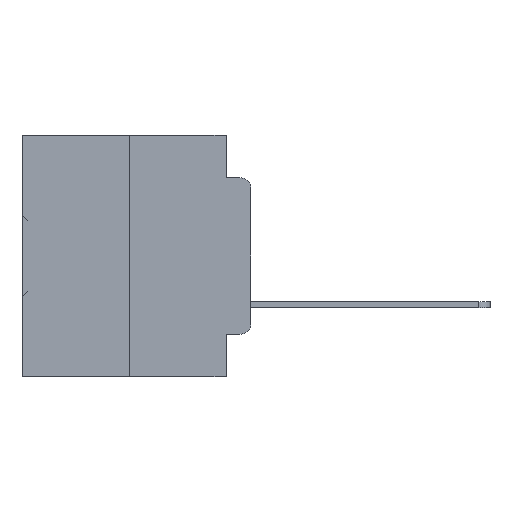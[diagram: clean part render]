
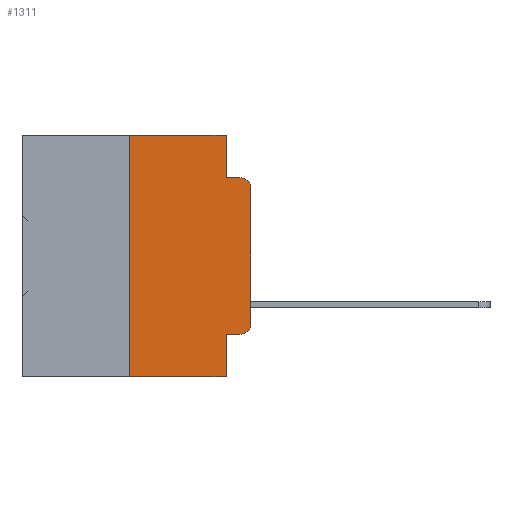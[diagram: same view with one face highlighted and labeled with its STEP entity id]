
A CAD part, left-side view. The second image highlights one B-rep face of the part: STEP entity #1311.
In plain terms, the highlighted planar face has unit normal (-1, 0, 0).
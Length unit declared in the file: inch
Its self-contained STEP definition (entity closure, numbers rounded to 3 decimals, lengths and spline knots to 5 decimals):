
#771 = EDGE_CURVE ( 'NONE', #20657, #15673, #15072, .T. ) ;
#1311 = ADVANCED_FACE ( 'NONE', ( #11215 ), #8687, .F. ) ;
#1824 = LINE ( 'NONE', #27525, #25090 ) ;
#2184 = VECTOR ( 'NONE', #33086, 39.37008 ) ;
#2272 = CARTESIAN_POINT ( 'NONE',  ( 0., 0.051, -0.4115 ) ) ;
#2706 = CARTESIAN_POINT ( 'NONE',  ( 0., 0.051, 0. ) ) ;
#3140 = ORIENTED_EDGE ( 'NONE', *, *, #29928, .T. ) ;
#3907 = VERTEX_POINT ( 'NONE', #31514 ) ;
#4711 = VERTEX_POINT ( 'NONE', #8743 ) ;
#5124 = CARTESIAN_POINT ( 'NONE',  ( 0., 0., -0.1085 ) ) ;
#5289 = CARTESIAN_POINT ( 'NONE',  ( 0., 0.02, -0.1085 ) ) ;
#5407 = ORIENTED_EDGE ( 'NONE', *, *, #12841, .F. ) ;
#5420 = ORIENTED_EDGE ( 'NONE', *, *, #36283, .F. ) ;
#6996 = VECTOR ( 'NONE', #14801, 39.37008 ) ;
#7180 = VECTOR ( 'NONE', #24824, 39.37008 ) ;
#7764 = EDGE_CURVE ( 'NONE', #3907, #27670, #10228, .T. ) ;
#8336 = DIRECTION ( 'NONE',  ( 0., 0., -1. ) ) ;
#8360 = LINE ( 'NONE', #26220, #14506 ) ;
#8659 = ORIENTED_EDGE ( 'NONE', *, *, #31378, .T. ) ;
#8687 = PLANE ( 'NONE',  #10043 ) ;
#8743 = CARTESIAN_POINT ( 'NONE',  ( 0., 0.02, -0.0885 ) ) ;
#9107 = DIRECTION ( 'NONE',  ( 0., -1., 0. ) ) ;
#9382 = VERTEX_POINT ( 'NONE', #32377 ) ;
#9793 = CARTESIAN_POINT ( 'NONE',  ( 0., 0.051, -0.0885 ) ) ;
#10043 = AXIS2_PLACEMENT_3D ( 'NONE', #36058, #17841, #39101 ) ;
#10228 = LINE ( 'NONE', #2706, #2184 ) ;
#11196 = CIRCLE ( 'NONE', #31931, 0.02 ) ;
#11215 = FACE_OUTER_BOUND ( 'NONE', #35360, .T. ) ;
#12841 = EDGE_CURVE ( 'NONE', #13925, #3907, #30212, .T. ) ;
#13925 = VERTEX_POINT ( 'NONE', #16389 ) ;
#14410 = CARTESIAN_POINT ( 'NONE',  ( 0., 0.02, -0.4115 ) ) ;
#14506 = VECTOR ( 'NONE', #20110, 39.37008 ) ;
#14801 = DIRECTION ( 'NONE',  ( 0., 0., -1. ) ) ;
#15072 = LINE ( 'NONE', #26926, #6996 ) ;
#15083 = CARTESIAN_POINT ( 'NONE',  ( 0., 0.473, -0.5 ) ) ;
#15673 = VERTEX_POINT ( 'NONE', #33550 ) ;
#16389 = CARTESIAN_POINT ( 'NONE',  ( 0., 0.25, 0. ) ) ;
#16732 = AXIS2_PLACEMENT_3D ( 'NONE', #35150, #16921, #38180 ) ;
#16921 = DIRECTION ( 'NONE',  ( -1., 0., 0. ) ) ;
#17728 = EDGE_CURVE ( 'NONE', #9382, #21263, #1824, .T. ) ;
#17841 = DIRECTION ( 'NONE',  ( 1., 0., 0. ) ) ;
#18744 = ORIENTED_EDGE ( 'NONE', *, *, #18811, .F. ) ;
#18811 = EDGE_CURVE ( 'NONE', #24144, #13925, #8360, .T. ) ;
#20110 = DIRECTION ( 'NONE',  ( 0., 0., 1. ) ) ;
#20512 = DIRECTION ( 'NONE',  ( 0., -1., 0. ) ) ;
#20615 = VECTOR ( 'NONE', #22107, 39.37008 ) ;
#20657 = VERTEX_POINT ( 'NONE', #2272 ) ;
#21263 = VERTEX_POINT ( 'NONE', #5124 ) ;
#21913 = CIRCLE ( 'NONE', #16732, 0.02 ) ;
#22107 = DIRECTION ( 'NONE',  ( 0., -1., 0. ) ) ;
#24144 = VERTEX_POINT ( 'NONE', #24286 ) ;
#24286 = CARTESIAN_POINT ( 'NONE',  ( 0., 0.25, -0.5 ) ) ;
#24824 = DIRECTION ( 'NONE',  ( 0., -1., 0. ) ) ;
#25090 = VECTOR ( 'NONE', #33464, 39.37008 ) ;
#25249 = LINE ( 'NONE', #9793, #7180 ) ;
#26220 = CARTESIAN_POINT ( 'NONE',  ( 0., 0.25, 0. ) ) ;
#26548 = DIRECTION ( 'NONE',  ( -1., 0., 0. ) ) ;
#26926 = CARTESIAN_POINT ( 'NONE',  ( 0., 0.051, 0. ) ) ;
#27014 = LINE ( 'NONE', #15083, #34129 ) ;
#27126 = ORIENTED_EDGE ( 'NONE', *, *, #17728, .T. ) ;
#27525 = CARTESIAN_POINT ( 'NONE',  ( 0., 0., 0. ) ) ;
#27670 = VERTEX_POINT ( 'NONE', #31642 ) ;
#28450 = EDGE_CURVE ( 'NONE', #21263, #4711, #11196, .T. ) ;
#28690 = LINE ( 'NONE', #31278, #20615 ) ;
#29208 = ORIENTED_EDGE ( 'NONE', *, *, #771, .F. ) ;
#29514 = ORIENTED_EDGE ( 'NONE', *, *, #28450, .T. ) ;
#29928 = EDGE_CURVE ( 'NONE', #20657, #34858, #28690, .T. ) ;
#30212 = LINE ( 'NONE', #32440, #36391 ) ;
#31278 = CARTESIAN_POINT ( 'NONE',  ( 0., 0.051, -0.4115 ) ) ;
#31378 = EDGE_CURVE ( 'NONE', #34858, #9382, #21913, .T. ) ;
#31514 = CARTESIAN_POINT ( 'NONE',  ( 0., 0.051, 0. ) ) ;
#31642 = CARTESIAN_POINT ( 'NONE',  ( 0., 0.051, -0.0885 ) ) ;
#31931 = AXIS2_PLACEMENT_3D ( 'NONE', #5289, #26548, #8336 ) ;
#32377 = CARTESIAN_POINT ( 'NONE',  ( 0., 0., -0.3915 ) ) ;
#32440 = CARTESIAN_POINT ( 'NONE',  ( 0., 0.473, 0. ) ) ;
#32758 = EDGE_CURVE ( 'NONE', #24144, #15673, #27014, .T. ) ;
#32769 = ORIENTED_EDGE ( 'NONE', *, *, #7764, .F. ) ;
#33086 = DIRECTION ( 'NONE',  ( 0., 0., -1. ) ) ;
#33464 = DIRECTION ( 'NONE',  ( 0., 0., 1. ) ) ;
#33550 = CARTESIAN_POINT ( 'NONE',  ( 0., 0.051, -0.5 ) ) ;
#34129 = VECTOR ( 'NONE', #9107, 39.37008 ) ;
#34757 = ORIENTED_EDGE ( 'NONE', *, *, #32758, .T. ) ;
#34858 = VERTEX_POINT ( 'NONE', #14410 ) ;
#35150 = CARTESIAN_POINT ( 'NONE',  ( 0., 0.02, -0.3915 ) ) ;
#35360 = EDGE_LOOP ( 'NONE', ( #27126, #29514, #5420, #32769, #5407, #18744, #34757, #29208, #3140, #8659 ) ) ;
#36058 = CARTESIAN_POINT ( 'NONE',  ( 0., 0.473, 0. ) ) ;
#36283 = EDGE_CURVE ( 'NONE', #27670, #4711, #25249, .T. ) ;
#36391 = VECTOR ( 'NONE', #20512, 39.37008 ) ;
#38180 = DIRECTION ( 'NONE',  ( 0., 0., -1. ) ) ;
#39101 = DIRECTION ( 'NONE',  ( 0., 0., -1. ) ) ;
